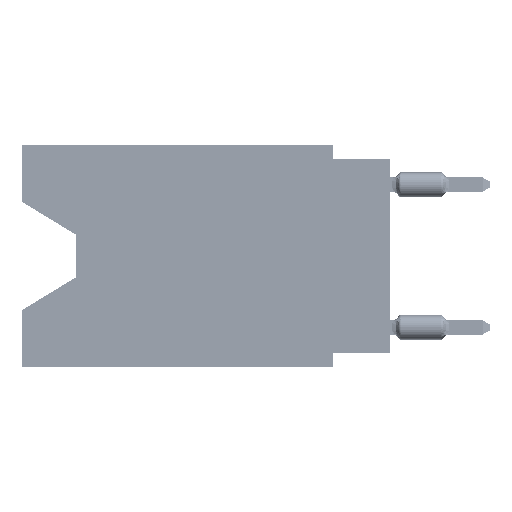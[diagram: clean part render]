
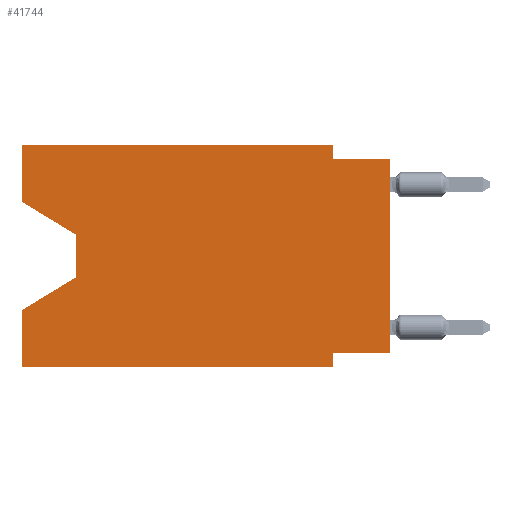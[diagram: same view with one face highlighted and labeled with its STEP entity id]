
A CAD part, left-side view. The second image highlights one B-rep face of the part: STEP entity #41744.
In plain terms, the highlighted planar face has unit normal (-1, 0, 0).
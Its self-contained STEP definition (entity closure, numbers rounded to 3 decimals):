
#196 = DIRECTION ( 'NONE',  ( 0., 0., 1. ) ) ;
#212 = VERTEX_POINT ( 'NONE', #41389 ) ;
#2564 = EDGE_CURVE ( 'NONE', #23717, #50410, #68915, .T. ) ;
#2599 = PLANE ( 'NONE',  #21137 ) ;
#3607 = CARTESIAN_POINT ( 'NONE',  ( 0., 2.54, 0. ) ) ;
#3946 = DIRECTION ( 'NONE',  ( 0., 0., -1. ) ) ;
#5444 = CARTESIAN_POINT ( 'NONE',  ( 0., 13.97, -5.893 ) ) ;
#5727 = DIRECTION ( 'NONE',  ( 0., 1., 0. ) ) ;
#5964 = ORIENTED_EDGE ( 'NONE', *, *, #64909, .T. ) ;
#6004 = VERTEX_POINT ( 'NONE', #39901 ) ;
#6058 = VECTOR ( 'NONE', #66739, 1000. ) ;
#6179 = LINE ( 'NONE', #34493, #61189 ) ;
#6327 = CARTESIAN_POINT ( 'NONE',  ( 0., 16.383, -9.906 ) ) ;
#6625 = LINE ( 'NONE', #13509, #26705 ) ;
#7149 = ORIENTED_EDGE ( 'NONE', *, *, #12651, .F. ) ;
#12651 = EDGE_CURVE ( 'NONE', #212, #67261, #45175, .T. ) ;
#12996 = VERTEX_POINT ( 'NONE', #83928 ) ;
#13509 = CARTESIAN_POINT ( 'NONE',  ( 0., 0., -9.271 ) ) ;
#14478 = DIRECTION ( 'NONE',  ( 0., -0.855, -0.519 ) ) ;
#16049 = EDGE_CURVE ( 'NONE', #78658, #212, #79696, .T. ) ;
#17235 = VERTEX_POINT ( 'NONE', #37196 ) ;
#18901 = EDGE_CURVE ( 'NONE', #67261, #70762, #37572, .T. ) ;
#20255 = ORIENTED_EDGE ( 'NONE', *, *, #18901, .F. ) ;
#21137 = AXIS2_PLACEMENT_3D ( 'NONE', #30007, #31823, #3946 ) ;
#23443 = ORIENTED_EDGE ( 'NONE', *, *, #16049, .F. ) ;
#23556 = CARTESIAN_POINT ( 'NONE',  ( 0., 0., -0.635 ) ) ;
#23717 = VERTEX_POINT ( 'NONE', #34324 ) ;
#24347 = ORIENTED_EDGE ( 'NONE', *, *, #2564, .T. ) ;
#26705 = VECTOR ( 'NONE', #5727, 1000. ) ;
#27282 = CARTESIAN_POINT ( 'NONE',  ( 0., 16.383, -2.546 ) ) ;
#28278 = LINE ( 'NONE', #78906, #46182 ) ;
#28980 = VERTEX_POINT ( 'NONE', #79518 ) ;
#29631 = CARTESIAN_POINT ( 'NONE',  ( 0., 2.54, -9.906 ) ) ;
#30007 = CARTESIAN_POINT ( 'NONE',  ( 0., 16.383, 0. ) ) ;
#30842 = VERTEX_POINT ( 'NONE', #46531 ) ;
#31823 = DIRECTION ( 'NONE',  ( 1., 0., 0. ) ) ;
#34048 = DIRECTION ( 'NONE',  ( 0., 0.855, -0.519 ) ) ;
#34324 = CARTESIAN_POINT ( 'NONE',  ( 0., 16.383, -9.906 ) ) ;
#34493 = CARTESIAN_POINT ( 'NONE',  ( 0., 13.97, -5.893 ) ) ;
#36001 = DIRECTION ( 'NONE',  ( 0., 0., 1. ) ) ;
#36684 = ORIENTED_EDGE ( 'NONE', *, *, #50966, .T. ) ;
#37196 = CARTESIAN_POINT ( 'NONE',  ( 0., 16.383, -2.546 ) ) ;
#37390 = VECTOR ( 'NONE', #74080, 1000. ) ;
#37572 = LINE ( 'NONE', #79583, #55214 ) ;
#37969 = CARTESIAN_POINT ( 'NONE',  ( 0., 13.97, -4.013 ) ) ;
#38031 = DIRECTION ( 'NONE',  ( 0., -1., 0. ) ) ;
#38311 = CARTESIAN_POINT ( 'NONE',  ( 0., 2.54, -9.906 ) ) ;
#39901 = CARTESIAN_POINT ( 'NONE',  ( 0., 16.383, -7.36 ) ) ;
#41064 = CARTESIAN_POINT ( 'NONE',  ( 0., 16.383, 0. ) ) ;
#41389 = CARTESIAN_POINT ( 'NONE',  ( 0., 2.54, 0. ) ) ;
#41744 = ADVANCED_FACE ( 'NONE', ( #44598 ), #2599, .F. ) ;
#43071 = CARTESIAN_POINT ( 'NONE',  ( 0., 0., 0. ) ) ;
#44598 = FACE_OUTER_BOUND ( 'NONE', #76538, .T. ) ;
#45175 = LINE ( 'NONE', #3607, #85049 ) ;
#46182 = VECTOR ( 'NONE', #36001, 1000. ) ;
#46531 = CARTESIAN_POINT ( 'NONE',  ( 0., 0., -9.271 ) ) ;
#46743 = VECTOR ( 'NONE', #196, 1000. ) ;
#46808 = ORIENTED_EDGE ( 'NONE', *, *, #63099, .F. ) ;
#49009 = LINE ( 'NONE', #62253, #83263 ) ;
#50410 = VERTEX_POINT ( 'NONE', #38311 ) ;
#50966 = EDGE_CURVE ( 'NONE', #55360, #6004, #6179, .T. ) ;
#54942 = DIRECTION ( 'NONE',  ( 0., 0., 1. ) ) ;
#55214 = VECTOR ( 'NONE', #38031, 1000. ) ;
#55360 = VERTEX_POINT ( 'NONE', #5444 ) ;
#56473 = EDGE_CURVE ( 'NONE', #17235, #78658, #28278, .T. ) ;
#56687 = VECTOR ( 'NONE', #63450, 1000. ) ;
#57192 = ORIENTED_EDGE ( 'NONE', *, *, #87143, .T. ) ;
#61189 = VECTOR ( 'NONE', #34048, 1000. ) ;
#62253 = CARTESIAN_POINT ( 'NONE',  ( 0., 16.383, 0. ) ) ;
#62766 = LINE ( 'NONE', #43071, #46743 ) ;
#63099 = EDGE_CURVE ( 'NONE', #23717, #6004, #49009, .T. ) ;
#63450 = DIRECTION ( 'NONE',  ( 0., 0., -1. ) ) ;
#64909 = EDGE_CURVE ( 'NONE', #30842, #70762, #62766, .T. ) ;
#65971 = EDGE_CURVE ( 'NONE', #28980, #55360, #85913, .T. ) ;
#66739 = DIRECTION ( 'NONE',  ( 0., 0., -1. ) ) ;
#67216 = CARTESIAN_POINT ( 'NONE',  ( 0., 2.54, -0.635 ) ) ;
#67261 = VERTEX_POINT ( 'NONE', #67216 ) ;
#68915 = LINE ( 'NONE', #6327, #37390 ) ;
#69853 = ORIENTED_EDGE ( 'NONE', *, *, #85226, .F. ) ;
#70196 = LINE ( 'NONE', #27282, #77166 ) ;
#70762 = VERTEX_POINT ( 'NONE', #23556 ) ;
#72078 = LINE ( 'NONE', #29631, #56687 ) ;
#74080 = DIRECTION ( 'NONE',  ( 0., -1., 0. ) ) ;
#76521 = EDGE_CURVE ( 'NONE', #30842, #12996, #6625, .T. ) ;
#76538 = EDGE_LOOP ( 'NONE', ( #57192, #83865, #36684, #46808, #24347, #69853, #89610, #5964, #20255, #7149, #23443, #78547 ) ) ;
#77166 = VECTOR ( 'NONE', #14478, 1000. ) ;
#78547 = ORIENTED_EDGE ( 'NONE', *, *, #56473, .F. ) ;
#78658 = VERTEX_POINT ( 'NONE', #41064 ) ;
#78906 = CARTESIAN_POINT ( 'NONE',  ( 0., 16.383, 0. ) ) ;
#79518 = CARTESIAN_POINT ( 'NONE',  ( 0., 13.97, -4.013 ) ) ;
#79583 = CARTESIAN_POINT ( 'NONE',  ( 0., 0., -0.635 ) ) ;
#79696 = LINE ( 'NONE', #87449, #79925 ) ;
#79925 = VECTOR ( 'NONE', #86543, 1000. ) ;
#83263 = VECTOR ( 'NONE', #54942, 1000. ) ;
#83865 = ORIENTED_EDGE ( 'NONE', *, *, #65971, .T. ) ;
#83928 = CARTESIAN_POINT ( 'NONE',  ( 0., 2.54, -9.271 ) ) ;
#85049 = VECTOR ( 'NONE', #85814, 1000. ) ;
#85226 = EDGE_CURVE ( 'NONE', #12996, #50410, #72078, .T. ) ;
#85814 = DIRECTION ( 'NONE',  ( 0., 0., -1. ) ) ;
#85913 = LINE ( 'NONE', #37969, #6058 ) ;
#86543 = DIRECTION ( 'NONE',  ( 0., -1., 0. ) ) ;
#87143 = EDGE_CURVE ( 'NONE', #17235, #28980, #70196, .T. ) ;
#87449 = CARTESIAN_POINT ( 'NONE',  ( 0., 16.383, 0. ) ) ;
#89610 = ORIENTED_EDGE ( 'NONE', *, *, #76521, .F. ) ;
